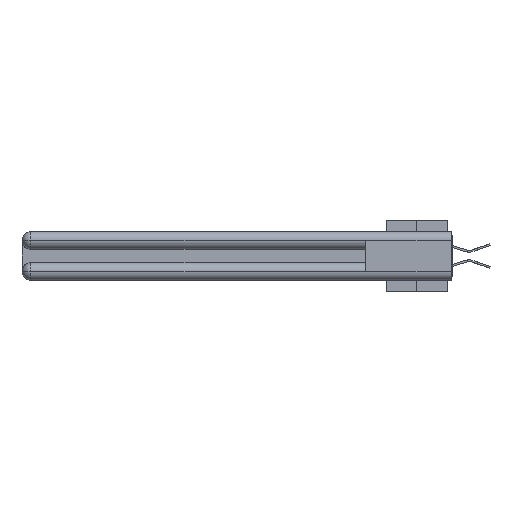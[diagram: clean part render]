
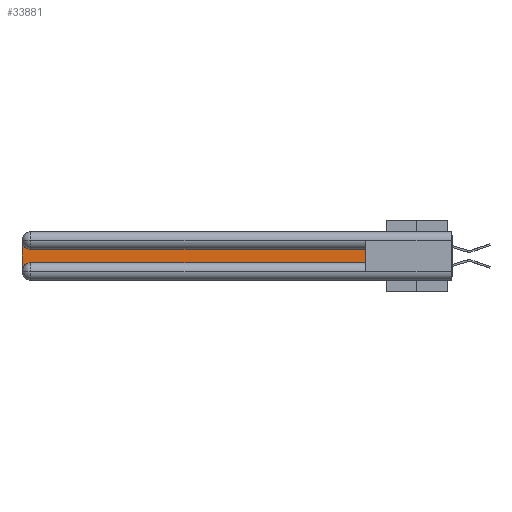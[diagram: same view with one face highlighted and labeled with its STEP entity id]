
A CAD part, left-side view. The second image highlights one B-rep face of the part: STEP entity #33881.
In plain terms, the highlighted planar face has unit normal (-1, 0, 0).
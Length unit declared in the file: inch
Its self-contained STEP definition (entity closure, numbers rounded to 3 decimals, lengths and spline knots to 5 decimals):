
#9 = CIRCLE ( 'NONE', #3553, 0.06 ) ;
#206 = LINE ( 'NONE', #20034, #16857 ) ;
#566 = LINE ( 'NONE', #25704, #35171 ) ;
#984 = EDGE_CURVE ( 'NONE', #21306, #33623, #206, .T. ) ;
#1668 = ORIENTED_EDGE ( 'NONE', *, *, #33601, .T. ) ;
#2009 = EDGE_CURVE ( 'NONE', #19440, #21306, #566, .T. ) ;
#3112 = LINE ( 'NONE', #22512, #30587 ) ;
#3553 = AXIS2_PLACEMENT_3D ( 'NONE', #8160, #31112, #36618 ) ;
#4501 = FACE_OUTER_BOUND ( 'NONE', #16036, .T. ) ;
#4849 = DIRECTION ( 'NONE',  ( 0., -1., 0. ) ) ;
#5110 = VERTEX_POINT ( 'NONE', #37190 ) ;
#6202 = CARTESIAN_POINT ( 'NONE',  ( 0.075, 0.6, -0.1225 ) ) ;
#6581 = EDGE_CURVE ( 'NONE', #29301, #36672, #3112, .T. ) ;
#8160 = CARTESIAN_POINT ( 'NONE',  ( 0.075, 2.94, -0.0625 ) ) ;
#8350 = EDGE_CURVE ( 'NONE', #5110, #19440, #20120, .T. ) ;
#11549 = DIRECTION ( 'NONE',  ( 0., 0., 1. ) ) ;
#11790 = PLANE ( 'NONE',  #24765 ) ;
#11929 = CARTESIAN_POINT ( 'NONE',  ( 0.075, 2.94, -0.2775 ) ) ;
#12463 = VECTOR ( 'NONE', #4849, 39.37008 ) ;
#14321 = CIRCLE ( 'NONE', #35679, 0.06 ) ;
#16036 = EDGE_LOOP ( 'NONE', ( #36133, #1668, #23082, #23115, #27512, #31369 ) ) ;
#16845 = CARTESIAN_POINT ( 'NONE',  ( 0.075, 3., -0.2775 ) ) ;
#16857 = VECTOR ( 'NONE', #22918, 39.37008 ) ;
#19440 = VERTEX_POINT ( 'NONE', #30814 ) ;
#20034 = CARTESIAN_POINT ( 'NONE',  ( 0.075, 0.6, -0.1225 ) ) ;
#20120 = LINE ( 'NONE', #30957, #12463 ) ;
#21306 = VERTEX_POINT ( 'NONE', #6202 ) ;
#22264 = DIRECTION ( 'NONE',  ( 0., 0., -1. ) ) ;
#22512 = CARTESIAN_POINT ( 'NONE',  ( 0.075, 3., -0.2175 ) ) ;
#22918 = DIRECTION ( 'NONE',  ( 0., 1., 0. ) ) ;
#23082 = ORIENTED_EDGE ( 'NONE', *, *, #6581, .T. ) ;
#23115 = ORIENTED_EDGE ( 'NONE', *, *, #29094, .T. ) ;
#23358 = DIRECTION ( 'NONE',  ( 0., 0., -1. ) ) ;
#23591 = DIRECTION ( 'NONE',  ( 1., 0., 0. ) ) ;
#24765 = AXIS2_PLACEMENT_3D ( 'NONE', #34735, #34617, #31979 ) ;
#25704 = CARTESIAN_POINT ( 'NONE',  ( 0.075, 0.6, -0.2175 ) ) ;
#27512 = ORIENTED_EDGE ( 'NONE', *, *, #8350, .T. ) ;
#29094 = EDGE_CURVE ( 'NONE', #36672, #5110, #14321, .T. ) ;
#29301 = VERTEX_POINT ( 'NONE', #30718 ) ;
#30587 = VECTOR ( 'NONE', #22264, 39.37008 ) ;
#30718 = CARTESIAN_POINT ( 'NONE',  ( 0.075, 3., -0.0625 ) ) ;
#30814 = CARTESIAN_POINT ( 'NONE',  ( 0.075, 0.6, -0.2175 ) ) ;
#30872 = CARTESIAN_POINT ( 'NONE',  ( 0.075, 2.94, -0.1225 ) ) ;
#30957 = CARTESIAN_POINT ( 'NONE',  ( 0.075, 0.6, -0.2175 ) ) ;
#31112 = DIRECTION ( 'NONE',  ( 1., 0., 0. ) ) ;
#31369 = ORIENTED_EDGE ( 'NONE', *, *, #2009, .T. ) ;
#31979 = DIRECTION ( 'NONE',  ( 0., 0., -1. ) ) ;
#33601 = EDGE_CURVE ( 'NONE', #33623, #29301, #9, .T. ) ;
#33623 = VERTEX_POINT ( 'NONE', #30872 ) ;
#33881 = ADVANCED_FACE ( 'NONE', ( #4501 ), #11790, .F. ) ;
#34617 = DIRECTION ( 'NONE',  ( 1., 0., 0. ) ) ;
#34735 = CARTESIAN_POINT ( 'NONE',  ( 0.075, 3., -0.1225 ) ) ;
#35171 = VECTOR ( 'NONE', #11549, 39.37008 ) ;
#35679 = AXIS2_PLACEMENT_3D ( 'NONE', #11929, #23591, #23358 ) ;
#36133 = ORIENTED_EDGE ( 'NONE', *, *, #984, .T. ) ;
#36618 = DIRECTION ( 'NONE',  ( 0., 0., -1. ) ) ;
#36672 = VERTEX_POINT ( 'NONE', #16845 ) ;
#37190 = CARTESIAN_POINT ( 'NONE',  ( 0.075, 2.94, -0.2175 ) ) ;
